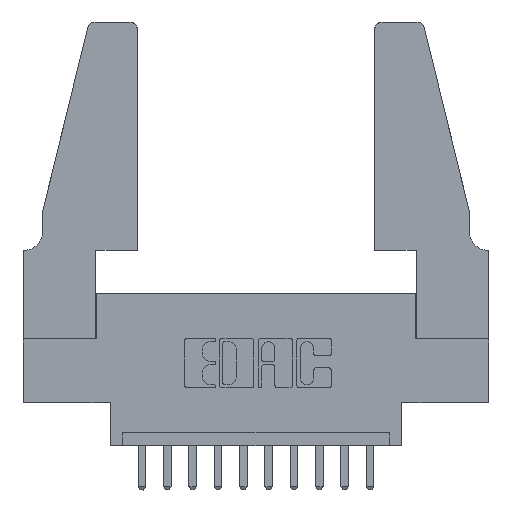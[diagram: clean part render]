
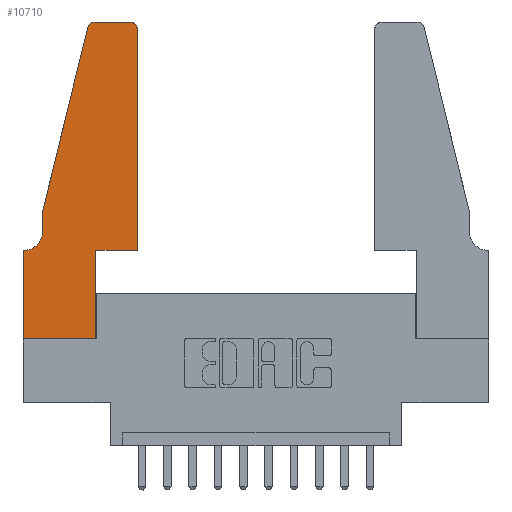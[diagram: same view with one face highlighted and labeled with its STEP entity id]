
A CAD part, top view. The second image highlights one B-rep face of the part: STEP entity #10710.
In plain terms, the highlighted planar face has unit normal (0, 0, 1).
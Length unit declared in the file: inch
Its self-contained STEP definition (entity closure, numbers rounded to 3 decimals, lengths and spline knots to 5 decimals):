
#23 = VERTEX_POINT ( 'NONE', #9725 ) ;
#29 = LINE ( 'NONE', #9188, #203 ) ;
#44 = CARTESIAN_POINT ( 'NONE',  ( 0.4205, 1.25, 0.37 ) ) ;
#72 = DIRECTION ( 'NONE',  ( 0., 0., 1. ) ) ;
#92 = AXIS2_PLACEMENT_3D ( 'NONE', #10984, #72, #7683 ) ;
#203 = VECTOR ( 'NONE', #2759, 39.37008 ) ;
#314 = CARTESIAN_POINT ( 'NONE',  ( 0.4505, 0.35, 0.37 ) ) ;
#369 = CARTESIAN_POINT ( 'NONE',  ( 0., 0., 0.37 ) ) ;
#389 = DIRECTION ( 'NONE',  ( 0., 0., 1. ) ) ;
#538 = CARTESIAN_POINT ( 'NONE',  ( 0., 0., 0.37 ) ) ;
#644 = VECTOR ( 'NONE', #8133, 39.37008 ) ;
#862 = EDGE_CURVE ( 'NONE', #5155, #3165, #2382, .T. ) ;
#989 = DIRECTION ( 'NONE',  ( -0.239, -0.971, 0. ) ) ;
#1084 = CARTESIAN_POINT ( 'NONE',  ( 0.0055, 0.42, 0.37 ) ) ;
#1158 = ORIENTED_EDGE ( 'NONE', *, *, #4138, .T. ) ;
#1171 = AXIS2_PLACEMENT_3D ( 'NONE', #5254, #1884, #7354 ) ;
#1324 = CARTESIAN_POINT ( 'NONE',  ( 0.0055, 0.35, 0.37 ) ) ;
#1584 = EDGE_CURVE ( 'NONE', #3165, #10128, #7442, .T. ) ;
#1611 = VERTEX_POINT ( 'NONE', #1849 ) ;
#1619 = CIRCLE ( 'NONE', #92, 0.03 ) ;
#1626 = VERTEX_POINT ( 'NONE', #11538 ) ;
#1797 = EDGE_CURVE ( 'NONE', #10128, #6068, #10540, .T. ) ;
#1815 = VERTEX_POINT ( 'NONE', #10251 ) ;
#1849 = CARTESIAN_POINT ( 'NONE',  ( 0.0755, 0.42, 0.37 ) ) ;
#1884 = DIRECTION ( 'NONE',  ( 0., 0., 1. ) ) ;
#2198 = CARTESIAN_POINT ( 'NONE',  ( 0.2865, 0.35, 0.37 ) ) ;
#2382 = LINE ( 'NONE', #14045, #10557 ) ;
#2394 = VECTOR ( 'NONE', #14183, 39.37008 ) ;
#2455 = ORIENTED_EDGE ( 'NONE', *, *, #1797, .T. ) ;
#2481 = ORIENTED_EDGE ( 'NONE', *, *, #3223, .T. ) ;
#2529 = CARTESIAN_POINT ( 'NONE',  ( 0.4505, 0.35, 0.37 ) ) ;
#2541 = DIRECTION ( 'NONE',  ( 1., 0., 0. ) ) ;
#2642 = LINE ( 'NONE', #8904, #4665 ) ;
#2743 = LINE ( 'NONE', #10846, #2394 ) ;
#2759 = DIRECTION ( 'NONE',  ( -1., 0., 0. ) ) ;
#2981 = ORIENTED_EDGE ( 'NONE', *, *, #11603, .T. ) ;
#3165 = VERTEX_POINT ( 'NONE', #314 ) ;
#3223 = EDGE_CURVE ( 'NONE', #5851, #9526, #1619, .T. ) ;
#3704 = EDGE_CURVE ( 'NONE', #7890, #23, #29, .T. ) ;
#3734 = EDGE_CURVE ( 'NONE', #1611, #7890, #3836, .T. ) ;
#3836 = CIRCLE ( 'NONE', #10121, 0.07 ) ;
#3981 = ORIENTED_EDGE ( 'NONE', *, *, #3704, .T. ) ;
#4107 = VECTOR ( 'NONE', #10404, 39.37008 ) ;
#4138 = EDGE_CURVE ( 'NONE', #1626, #5155, #2642, .T. ) ;
#4665 = VECTOR ( 'NONE', #12110, 39.37008 ) ;
#5155 = VERTEX_POINT ( 'NONE', #2198 ) ;
#5254 = CARTESIAN_POINT ( 'NONE',  ( 0., 0.35, 0.37 ) ) ;
#5330 = DIRECTION ( 'NONE',  ( 0., -1., 0. ) ) ;
#5562 = VECTOR ( 'NONE', #5330, 39.37008 ) ;
#5662 = CARTESIAN_POINT ( 'NONE',  ( 0.284, 1.25, 0.37 ) ) ;
#5851 = VERTEX_POINT ( 'NONE', #5662 ) ;
#6068 = VERTEX_POINT ( 'NONE', #44 ) ;
#6128 = ORIENTED_EDGE ( 'NONE', *, *, #7628, .T. ) ;
#6138 = ORIENTED_EDGE ( 'NONE', *, *, #11880, .T. ) ;
#6290 = ORIENTED_EDGE ( 'NONE', *, *, #1584, .T. ) ;
#6806 = LINE ( 'NONE', #369, #644 ) ;
#6880 = AXIS2_PLACEMENT_3D ( 'NONE', #12491, #389, #2541 ) ;
#7085 = LINE ( 'NONE', #11939, #5562 ) ;
#7119 = VECTOR ( 'NONE', #989, 39.37008 ) ;
#7354 = DIRECTION ( 'NONE',  ( 1., 0., 0. ) ) ;
#7442 = LINE ( 'NONE', #2529, #9164 ) ;
#7628 = EDGE_CURVE ( 'NONE', #9526, #7730, #10053, .T. ) ;
#7683 = DIRECTION ( 'NONE',  ( 1., 0., 0. ) ) ;
#7730 = VERTEX_POINT ( 'NONE', #11806 ) ;
#7890 = VERTEX_POINT ( 'NONE', #1324 ) ;
#8133 = DIRECTION ( 'NONE',  ( 0., -1., 0. ) ) ;
#8382 = CARTESIAN_POINT ( 'NONE',  ( 0.0755, 0.5, 0.37 ) ) ;
#8390 = CARTESIAN_POINT ( 'NONE',  ( 0.25487, 1.22718, 0.37 ) ) ;
#8665 = DIRECTION ( 'NONE',  ( 0., 0., -1. ) ) ;
#8904 = CARTESIAN_POINT ( 'NONE',  ( 0.2865, 0.35, 0.37 ) ) ;
#9164 = VECTOR ( 'NONE', #13474, 39.37008 ) ;
#9188 = CARTESIAN_POINT ( 'NONE',  ( 0.0755, 0.35, 0.37 ) ) ;
#9526 = VERTEX_POINT ( 'NONE', #8390 ) ;
#9630 = ORIENTED_EDGE ( 'NONE', *, *, #862, .T. ) ;
#9725 = CARTESIAN_POINT ( 'NONE',  ( 0., 0.35, 0.37 ) ) ;
#10053 = LINE ( 'NONE', #8382, #7119 ) ;
#10121 = AXIS2_PLACEMENT_3D ( 'NONE', #1084, #8665, #13016 ) ;
#10128 = VERTEX_POINT ( 'NONE', #11361 ) ;
#10251 = CARTESIAN_POINT ( 'NONE',  ( 0., 0., 0.37 ) ) ;
#10273 = FACE_OUTER_BOUND ( 'NONE', #13169, .T. ) ;
#10404 = DIRECTION ( 'NONE',  ( 1., 0., 0. ) ) ;
#10411 = LINE ( 'NONE', #538, #4107 ) ;
#10460 = DIRECTION ( 'NONE',  ( 1., 0., 0. ) ) ;
#10540 = CIRCLE ( 'NONE', #6880, 0.03 ) ;
#10557 = VECTOR ( 'NONE', #10460, 39.37008 ) ;
#10676 = ORIENTED_EDGE ( 'NONE', *, *, #3734, .T. ) ;
#10710 = ADVANCED_FACE ( 'NONE', ( #10273 ), #11855, .T. ) ;
#10846 = CARTESIAN_POINT ( 'NONE',  ( 0.2605, 1.25, 0.37 ) ) ;
#10984 = CARTESIAN_POINT ( 'NONE',  ( 0.284, 1.22, 0.37 ) ) ;
#11308 = EDGE_CURVE ( 'NONE', #1815, #1626, #10411, .T. ) ;
#11361 = CARTESIAN_POINT ( 'NONE',  ( 0.4505, 1.22, 0.37 ) ) ;
#11538 = CARTESIAN_POINT ( 'NONE',  ( 0.2865, 0., 0.37 ) ) ;
#11603 = EDGE_CURVE ( 'NONE', #6068, #5851, #2743, .T. ) ;
#11806 = CARTESIAN_POINT ( 'NONE',  ( 0.0755, 0.5, 0.37 ) ) ;
#11855 = PLANE ( 'NONE',  #1171 ) ;
#11880 = EDGE_CURVE ( 'NONE', #23, #1815, #6806, .T. ) ;
#11939 = CARTESIAN_POINT ( 'NONE',  ( 0.0755, 0.5, 0.37 ) ) ;
#12110 = DIRECTION ( 'NONE',  ( 0., 1., 0. ) ) ;
#12491 = CARTESIAN_POINT ( 'NONE',  ( 0.4205, 1.22, 0.37 ) ) ;
#13016 = DIRECTION ( 'NONE',  ( -1., 0., 0. ) ) ;
#13169 = EDGE_LOOP ( 'NONE', ( #2981, #2481, #6128, #13419, #10676, #3981, #6138, #13252, #1158, #9630, #6290, #2455 ) ) ;
#13252 = ORIENTED_EDGE ( 'NONE', *, *, #11308, .T. ) ;
#13419 = ORIENTED_EDGE ( 'NONE', *, *, #13920, .T. ) ;
#13474 = DIRECTION ( 'NONE',  ( 0., 1., 0. ) ) ;
#13920 = EDGE_CURVE ( 'NONE', #7730, #1611, #7085, .T. ) ;
#14045 = CARTESIAN_POINT ( 'NONE',  ( 0.4505, 0.35, 0.37 ) ) ;
#14183 = DIRECTION ( 'NONE',  ( -1., 0., 0. ) ) ;
